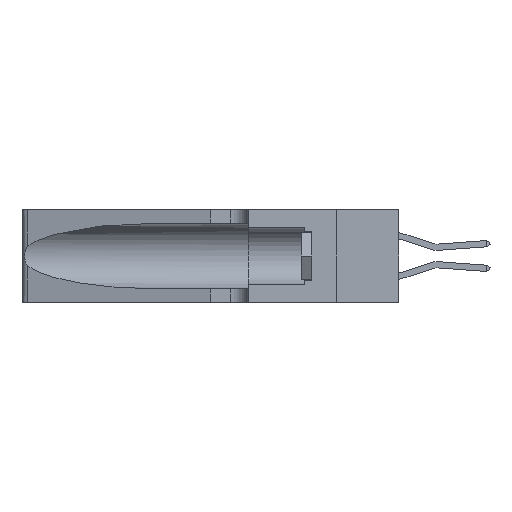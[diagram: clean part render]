
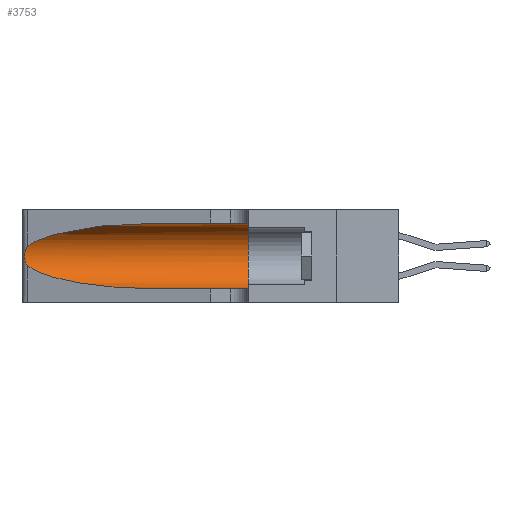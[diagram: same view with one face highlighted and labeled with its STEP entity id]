
A CAD part, left-side view. The second image highlights one B-rep face of the part: STEP entity #3753.
In plain terms, the highlighted cylindrical face has radius 3.308 mm (diameter 6.617 mm), a partial arc.
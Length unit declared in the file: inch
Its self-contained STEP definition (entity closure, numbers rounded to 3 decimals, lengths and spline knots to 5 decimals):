
#590 = CIRCLE ( 'NONE', #13260, 0.13025 ) ;
#638 = CARTESIAN_POINT ( 'NONE',  ( 0.2373, 1.15595, 0.08982 ) ) ;
#1180 = CARTESIAN_POINT ( 'NONE',  ( 0.26018, 1.23835, 0.19895 ) ) ;
#1406 = VECTOR ( 'NONE', #13460, 39.37008 ) ;
#1479 = CARTESIAN_POINT ( 'NONE',  ( 0.25487, 1.22718, 0.22369 ) ) ;
#1892 = ORIENTED_EDGE ( 'NONE', *, *, #11422, .T. ) ;
#2780 = CARTESIAN_POINT ( 'NONE',  ( 0.26075, 1.23896, 0.178 ) ) ;
#3373 = DIRECTION ( 'NONE',  ( 0., 1., 0. ) ) ;
#3753 = ADVANCED_FACE ( 'NONE', ( #16096 ), #8226, .F. ) ;
#4095 = ORIENTED_EDGE ( 'NONE', *, *, #11278, .T. ) ;
#4819 = VECTOR ( 'NONE', #6349, 39.37008 ) ;
#5255 = CARTESIAN_POINT ( 'NONE',  ( 0.1305, 0.35, 0.185 ) ) ;
#5818 = LINE ( 'NONE', #15071, #4819 ) ;
#6018 = VERTEX_POINT ( 'NONE', #12942 ) ;
#6104 = VERTEX_POINT ( 'NONE', #20313 ) ;
#6107 = CARTESIAN_POINT ( 'NONE',  ( 0.25487, 1.22718, 0.14631 ) ) ;
#6267 = CARTESIAN_POINT ( 'NONE',  ( 0.25639, 1.23184, 0.21858 ) ) ;
#6349 = DIRECTION ( 'NONE',  ( 0., -1., 0. ) ) ;
#6554 = VERTEX_POINT ( 'NONE', #18927 ) ;
#6576 = CARTESIAN_POINT ( 'NONE',  ( 0.1305, 0.72297, 0.31525 ) ) ;
#7253 = ORIENTED_EDGE ( 'NONE', *, *, #14458, .F. ) ;
#7679 = CARTESIAN_POINT ( 'NONE',  ( 0.25789, 1.23486, 0.15765 ) ) ;
#8034 = VERTEX_POINT ( 'NONE', #12871 ) ;
#8113 = EDGE_LOOP ( 'NONE', ( #4095, #18979, #1892, #16966, #12712, #7253 ) ) ;
#8226 = CYLINDRICAL_SURFACE ( 'NONE', #15348, 0.13025 ) ;
#8336 = CARTESIAN_POINT ( 'NONE',  ( 0.1305, 1.61858, 0.185 ) ) ;
#9828 = DIRECTION ( 'NONE',  ( 0., -1., 0. ) ) ;
#9958 = CARTESIAN_POINT ( 'NONE',  ( 0.25487, 1.22718, 0.22369 ) ) ;
#10786 = CARTESIAN_POINT ( 'NONE',  ( 0.26075, 1.23896, 0.19203 ) ) ;
#11278 = EDGE_CURVE ( 'NONE', #19629, #6104, #13445, .T. ) ;
#11422 = EDGE_CURVE ( 'NONE', #17793, #6554, #17890, .T. ) ;
#11797 = CARTESIAN_POINT ( 'NONE',  ( 0.18966, 0.96281, 0.05475 ) ) ;
#12423 = LINE ( 'NONE', #14947, #1406 ) ;
#12470 = CARTESIAN_POINT ( 'NONE',  ( 0.25856, 1.23593, 0.16098 ) ) ;
#12689 = CARTESIAN_POINT ( 'NONE',  ( 0.25555, 1.22994, 0.2215 ) ) ;
#12712 = ORIENTED_EDGE ( 'NONE', *, *, #16333, .F. ) ;
#12871 = CARTESIAN_POINT ( 'NONE',  ( 0.1305, 0.35, 0.05475 ) ) ;
#12942 = CARTESIAN_POINT ( 'NONE',  ( 0.1305, 0.35, 0.31525 ) ) ;
#13087 = DIRECTION ( 'NONE',  ( 0., 0., 1. ) ) ;
#13260 = AXIS2_PLACEMENT_3D ( 'NONE', #5255, #3373, #13087 ) ;
#13445 =( BOUNDED_CURVE ( )  B_SPLINE_CURVE ( 3, ( #6576, #19708, #16516, #9958 ),
 .UNSPECIFIED., .F., .F. ) 
 B_SPLINE_CURVE_WITH_KNOTS ( ( 4, 4 ),
 ( 1.5708, 2.84003 ),
 .UNSPECIFIED. ) 
 CURVE ( )  GEOMETRIC_REPRESENTATION_ITEM ( )  RATIONAL_B_SPLINE_CURVE ( ( 1., 0.87, 0.87, 1. ) ) 
 REPRESENTATION_ITEM ( '' )  );
#13460 = DIRECTION ( 'NONE',  ( 0., -1., 0. ) ) ;
#13660 = CARTESIAN_POINT ( 'NONE',  ( 0.25487, 1.22718, 0.14631 ) ) ;
#13907 = EDGE_CURVE ( 'NONE', #6104, #17793, #14108, .T. ) ;
#14108 = B_SPLINE_CURVE_WITH_KNOTS ( 'NONE', 3,
 ( #1479, #12689, #6267, #14352, #18882, #1180, #10786, #2780, #18959, #12470, #7679, #15754, #17402, #19037 ),
 .UNSPECIFIED., .F., .F.,
 ( 4, 2, 2, 2, 2, 2, 4 ),
 ( 0., 0.00027, 0.00053, 0.00107, 0.0016, 0.00187, 0.00214 ),
 .UNSPECIFIED. ) ;
#14352 = CARTESIAN_POINT ( 'NONE',  ( 0.25787, 1.23484, 0.2124 ) ) ;
#14383 = CARTESIAN_POINT ( 'NONE',  ( 0.1305, 0.72297, 0.31525 ) ) ;
#14458 = EDGE_CURVE ( 'NONE', #19629, #6018, #12423, .T. ) ;
#14947 = CARTESIAN_POINT ( 'NONE',  ( 0.1305, 1.61858, 0.31525 ) ) ;
#15071 = CARTESIAN_POINT ( 'NONE',  ( 0.1305, 1.61858, 0.05475 ) ) ;
#15348 = AXIS2_PLACEMENT_3D ( 'NONE', #8336, #9828, #16455 ) ;
#15754 = CARTESIAN_POINT ( 'NONE',  ( 0.25639, 1.23186, 0.15144 ) ) ;
#16096 = FACE_OUTER_BOUND ( 'NONE', #8113, .T. ) ;
#16333 = EDGE_CURVE ( 'NONE', #6018, #8034, #590, .T. ) ;
#16455 = DIRECTION ( 'NONE',  ( 0., 0., -1. ) ) ;
#16516 = CARTESIAN_POINT ( 'NONE',  ( 0.2373, 1.15595, 0.28018 ) ) ;
#16931 = CARTESIAN_POINT ( 'NONE',  ( 0.1305, 0.72297, 0.05475 ) ) ;
#16945 = EDGE_CURVE ( 'NONE', #6554, #8034, #5818, .T. ) ;
#16966 = ORIENTED_EDGE ( 'NONE', *, *, #16945, .T. ) ;
#17402 = CARTESIAN_POINT ( 'NONE',  ( 0.25555, 1.22993, 0.14849 ) ) ;
#17793 = VERTEX_POINT ( 'NONE', #6107 ) ;
#17890 =( BOUNDED_CURVE ( )  B_SPLINE_CURVE ( 3, ( #13660, #638, #11797, #16931 ),
 .UNSPECIFIED., .F., .F. ) 
 B_SPLINE_CURVE_WITH_KNOTS ( ( 4, 4 ),
 ( 3.44316, 4.71239 ),
 .UNSPECIFIED. ) 
 CURVE ( )  GEOMETRIC_REPRESENTATION_ITEM ( )  RATIONAL_B_SPLINE_CURVE ( ( 1., 0.87, 0.87, 1. ) ) 
 REPRESENTATION_ITEM ( '' )  );
#18882 = CARTESIAN_POINT ( 'NONE',  ( 0.25854, 1.2359, 0.20912 ) ) ;
#18927 = CARTESIAN_POINT ( 'NONE',  ( 0.1305, 0.72297, 0.05475 ) ) ;
#18959 = CARTESIAN_POINT ( 'NONE',  ( 0.26017, 1.23833, 0.17102 ) ) ;
#18979 = ORIENTED_EDGE ( 'NONE', *, *, #13907, .T. ) ;
#19037 = CARTESIAN_POINT ( 'NONE',  ( 0.25487, 1.22718, 0.14631 ) ) ;
#19629 = VERTEX_POINT ( 'NONE', #14383 ) ;
#19708 = CARTESIAN_POINT ( 'NONE',  ( 0.18966, 0.96281, 0.31525 ) ) ;
#20313 = CARTESIAN_POINT ( 'NONE',  ( 0.25487, 1.22718, 0.22369 ) ) ;
